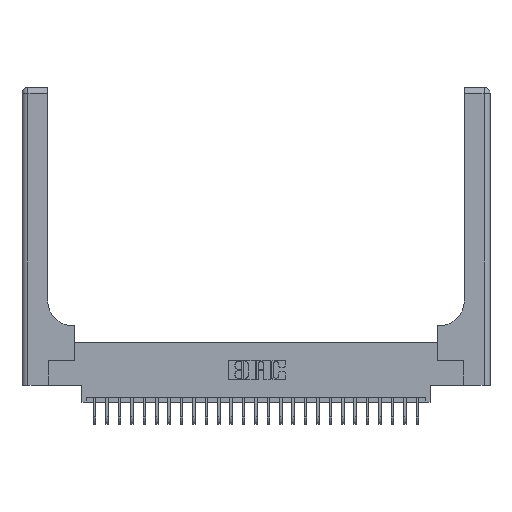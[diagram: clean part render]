
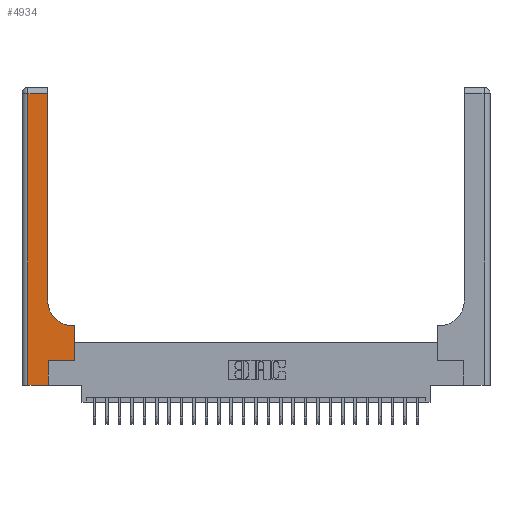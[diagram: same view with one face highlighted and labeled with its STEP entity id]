
A CAD part, top view. The second image highlights one B-rep face of the part: STEP entity #4934.
In plain terms, the highlighted planar face has unit normal (0, 0, 1).
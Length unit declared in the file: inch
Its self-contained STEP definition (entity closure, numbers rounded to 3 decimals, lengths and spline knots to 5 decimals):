
#11 = ORIENTED_EDGE ( 'NONE', *, *, #22674, .T. ) ;
#158 = VERTEX_POINT ( 'NONE', #20565 ) ;
#583 = ORIENTED_EDGE ( 'NONE', *, *, #22856, .T. ) ;
#941 = DIRECTION ( 'NONE',  ( -1., 0., 0. ) ) ;
#1012 = FACE_OUTER_BOUND ( 'NONE', #11311, .T. ) ;
#1159 = DIRECTION ( 'NONE',  ( -1., 0., 0. ) ) ;
#1433 = DIRECTION ( 'NONE',  ( 1., 0., 0. ) ) ;
#1975 = VECTOR ( 'NONE', #19492, 39.37008 ) ;
#2549 = LINE ( 'NONE', #19631, #1975 ) ;
#2880 = ORIENTED_EDGE ( 'NONE', *, *, #23071, .T. ) ;
#3275 = VECTOR ( 'NONE', #6278, 39.37008 ) ;
#3317 = VECTOR ( 'NONE', #25864, 39.37008 ) ;
#4013 = LINE ( 'NONE', #8540, #6330 ) ;
#4087 = DIRECTION ( 'NONE',  ( -1., 0., 0. ) ) ;
#4280 = VECTOR ( 'NONE', #11999, 39.37008 ) ;
#4934 = ADVANCED_FACE ( 'NONE', ( #1012 ), #17831, .F. ) ;
#5068 = LINE ( 'NONE', #13494, #10209 ) ;
#5545 = CARTESIAN_POINT ( 'NONE',  ( 0.51, 0.6, 0.37 ) ) ;
#5615 = EDGE_CURVE ( 'NONE', #25370, #158, #15878, .T. ) ;
#5880 = DIRECTION ( 'NONE',  ( 0., 1., 0. ) ) ;
#6245 = ORIENTED_EDGE ( 'NONE', *, *, #8458, .T. ) ;
#6278 = DIRECTION ( 'NONE',  ( 1., 0., 0. ) ) ;
#6330 = VECTOR ( 'NONE', #12678, 39.37008 ) ;
#6681 = CARTESIAN_POINT ( 'NONE',  ( 0.265, 0.25, 0.37 ) ) ;
#7614 = CARTESIAN_POINT ( 'NONE',  ( 0.06, 2.94, 0.37 ) ) ;
#7658 = VECTOR ( 'NONE', #4087, 39.37008 ) ;
#7952 = CARTESIAN_POINT ( 'NONE',  ( 0.26, 3., 0.37 ) ) ;
#8458 = EDGE_CURVE ( 'NONE', #13365, #22205, #26805, .T. ) ;
#8540 = CARTESIAN_POINT ( 'NONE',  ( 0., 0., 0.37 ) ) ;
#8705 = VERTEX_POINT ( 'NONE', #5545 ) ;
#9095 = ORIENTED_EDGE ( 'NONE', *, *, #10736, .T. ) ;
#9214 = AXIS2_PLACEMENT_3D ( 'NONE', #21648, #26204, #1159 ) ;
#9879 = CARTESIAN_POINT ( 'NONE',  ( 0.26, 0.6, 0.37 ) ) ;
#10209 = VECTOR ( 'NONE', #941, 39.37008 ) ;
#10377 = CARTESIAN_POINT ( 'NONE',  ( 0.26, 2.94, 0.37 ) ) ;
#10736 = EDGE_CURVE ( 'NONE', #22205, #23748, #5068, .T. ) ;
#11074 = LINE ( 'NONE', #6681, #3275 ) ;
#11311 = EDGE_LOOP ( 'NONE', ( #6245, #9095, #26550, #11, #15091, #2880, #13934, #583, #16868 ) ) ;
#11781 = EDGE_CURVE ( 'NONE', #8705, #13365, #23003, .T. ) ;
#11999 = DIRECTION ( 'NONE',  ( 0., 1., 0. ) ) ;
#12678 = DIRECTION ( 'NONE',  ( 1., 0., 0. ) ) ;
#13365 = VERTEX_POINT ( 'NONE', #22062 ) ;
#13494 = CARTESIAN_POINT ( 'NONE',  ( 0., 2.94, 0.37 ) ) ;
#13934 = ORIENTED_EDGE ( 'NONE', *, *, #15983, .T. ) ;
#15076 = AXIS2_PLACEMENT_3D ( 'NONE', #18385, #20297, #1433 ) ;
#15091 = ORIENTED_EDGE ( 'NONE', *, *, #5615, .T. ) ;
#15205 = VERTEX_POINT ( 'NONE', #18076 ) ;
#15878 = LINE ( 'NONE', #24261, #4280 ) ;
#15983 = EDGE_CURVE ( 'NONE', #15205, #26863, #2549, .T. ) ;
#15984 = CARTESIAN_POINT ( 'NONE',  ( 0.06, 3., 0.37 ) ) ;
#16539 = EDGE_CURVE ( 'NONE', #23748, #22497, #21591, .T. ) ;
#16868 = ORIENTED_EDGE ( 'NONE', *, *, #11781, .T. ) ;
#17831 = PLANE ( 'NONE',  #9214 ) ;
#18076 = CARTESIAN_POINT ( 'NONE',  ( 0.528, 0.25, 0.37 ) ) ;
#18193 = CARTESIAN_POINT ( 'NONE',  ( 0.528, 0.6, 0.37 ) ) ;
#18385 = CARTESIAN_POINT ( 'NONE',  ( 0.51, 0.85, 0.37 ) ) ;
#19492 = DIRECTION ( 'NONE',  ( 0., 1., 0. ) ) ;
#19631 = CARTESIAN_POINT ( 'NONE',  ( 0.528, 0.25, 0.37 ) ) ;
#20010 = CARTESIAN_POINT ( 'NONE',  ( 0.06, 0., 0.37 ) ) ;
#20297 = DIRECTION ( 'NONE',  ( 0., 0., -1. ) ) ;
#20565 = CARTESIAN_POINT ( 'NONE',  ( 0.265, 0.25, 0.37 ) ) ;
#21591 = LINE ( 'NONE', #15984, #3317 ) ;
#21648 = CARTESIAN_POINT ( 'NONE',  ( 0., 3., 0.37 ) ) ;
#22062 = CARTESIAN_POINT ( 'NONE',  ( 0.26, 0.85, 0.37 ) ) ;
#22205 = VERTEX_POINT ( 'NONE', #10377 ) ;
#22497 = VERTEX_POINT ( 'NONE', #20010 ) ;
#22674 = EDGE_CURVE ( 'NONE', #22497, #25370, #4013, .T. ) ;
#22856 = EDGE_CURVE ( 'NONE', #26863, #8705, #24486, .T. ) ;
#22875 = VECTOR ( 'NONE', #5880, 39.37008 ) ;
#23003 = CIRCLE ( 'NONE', #15076, 0.25 ) ;
#23071 = EDGE_CURVE ( 'NONE', #158, #15205, #11074, .T. ) ;
#23748 = VERTEX_POINT ( 'NONE', #7614 ) ;
#24261 = CARTESIAN_POINT ( 'NONE',  ( 0.265, 0., 0.37 ) ) ;
#24486 = LINE ( 'NONE', #9879, #7658 ) ;
#25370 = VERTEX_POINT ( 'NONE', #26972 ) ;
#25864 = DIRECTION ( 'NONE',  ( 0., -1., 0. ) ) ;
#26204 = DIRECTION ( 'NONE',  ( 0., 0., -1. ) ) ;
#26550 = ORIENTED_EDGE ( 'NONE', *, *, #16539, .T. ) ;
#26805 = LINE ( 'NONE', #7952, #22875 ) ;
#26863 = VERTEX_POINT ( 'NONE', #18193 ) ;
#26972 = CARTESIAN_POINT ( 'NONE',  ( 0.265, 0., 0.37 ) ) ;
